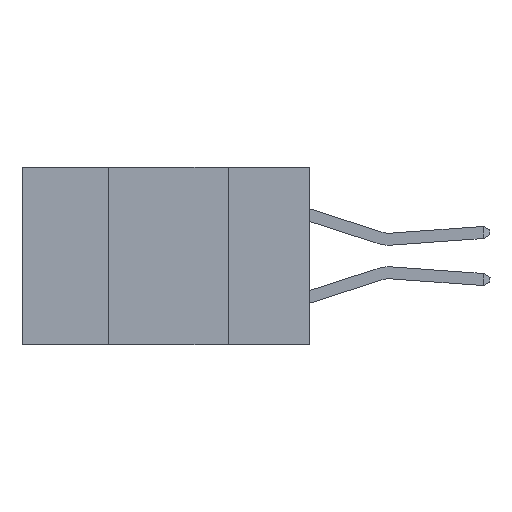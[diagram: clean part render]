
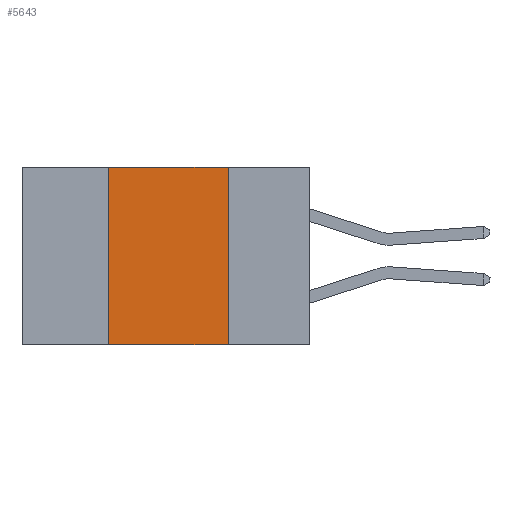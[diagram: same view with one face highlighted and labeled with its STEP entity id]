
A CAD part, left-side view. The second image highlights one B-rep face of the part: STEP entity #5643.
In plain terms, the highlighted planar face has unit normal (-1, 0, 0).
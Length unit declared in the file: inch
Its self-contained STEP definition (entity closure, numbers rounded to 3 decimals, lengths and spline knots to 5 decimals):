
#545 = VECTOR ( 'NONE', #7744, 39.37008 ) ;
#1086 = LINE ( 'NONE', #6898, #16368 ) ;
#1357 = DIRECTION ( 'NONE',  ( 1., 0., 0. ) ) ;
#2633 = LINE ( 'NONE', #10564, #545 ) ;
#2841 = FACE_OUTER_BOUND ( 'NONE', #14338, .T. ) ;
#2981 = AXIS2_PLACEMENT_3D ( 'NONE', #3991, #1357, #16227 ) ;
#3159 = VERTEX_POINT ( 'NONE', #8456 ) ;
#3181 = ORIENTED_EDGE ( 'NONE', *, *, #12433, .F. ) ;
#3991 = CARTESIAN_POINT ( 'NONE',  ( 0., 0.6, 0. ) ) ;
#4136 = VERTEX_POINT ( 'NONE', #11434 ) ;
#4713 = VECTOR ( 'NONE', #10268, 39.37008 ) ;
#4850 = VERTEX_POINT ( 'NONE', #12985 ) ;
#5612 = EDGE_CURVE ( 'NONE', #4136, #10545, #15207, .T. ) ;
#5643 = ADVANCED_FACE ( 'NONE', ( #2841 ), #8019, .F. ) ;
#5996 = CARTESIAN_POINT ( 'NONE',  ( 0., 0.17, -0.37 ) ) ;
#6898 = CARTESIAN_POINT ( 'NONE',  ( 0., 0.6, -0.37 ) ) ;
#7339 = ORIENTED_EDGE ( 'NONE', *, *, #5612, .F. ) ;
#7744 = DIRECTION ( 'NONE',  ( 0., 0., 1. ) ) ;
#7962 = EDGE_CURVE ( 'NONE', #4850, #10545, #1086, .T. ) ;
#8019 = PLANE ( 'NONE',  #2981 ) ;
#8456 = CARTESIAN_POINT ( 'NONE',  ( 0., 0.42, 0. ) ) ;
#8902 = CARTESIAN_POINT ( 'NONE',  ( 0., 0.6, 0. ) ) ;
#9320 = ORIENTED_EDGE ( 'NONE', *, *, #15902, .F. ) ;
#10268 = DIRECTION ( 'NONE',  ( 0., -1., 0. ) ) ;
#10545 = VERTEX_POINT ( 'NONE', #5996 ) ;
#10564 = CARTESIAN_POINT ( 'NONE',  ( 0., 0.42, 0. ) ) ;
#11304 = ORIENTED_EDGE ( 'NONE', *, *, #7962, .T. ) ;
#11434 = CARTESIAN_POINT ( 'NONE',  ( 0., 0.17, 0. ) ) ;
#11824 = LINE ( 'NONE', #8902, #4713 ) ;
#12433 = EDGE_CURVE ( 'NONE', #4850, #3159, #2633, .T. ) ;
#12878 = CARTESIAN_POINT ( 'NONE',  ( 0., 0.17, 0. ) ) ;
#12985 = CARTESIAN_POINT ( 'NONE',  ( 0., 0.42, -0.37 ) ) ;
#13537 = VECTOR ( 'NONE', #16899, 39.37008 ) ;
#14338 = EDGE_LOOP ( 'NONE', ( #7339, #9320, #3181, #11304 ) ) ;
#15207 = LINE ( 'NONE', #12878, #13537 ) ;
#15902 = EDGE_CURVE ( 'NONE', #3159, #4136, #11824, .T. ) ;
#16227 = DIRECTION ( 'NONE',  ( 0., 0., -1. ) ) ;
#16368 = VECTOR ( 'NONE', #16391, 39.37008 ) ;
#16391 = DIRECTION ( 'NONE',  ( 0., -1., 0. ) ) ;
#16899 = DIRECTION ( 'NONE',  ( 0., 0., -1. ) ) ;
